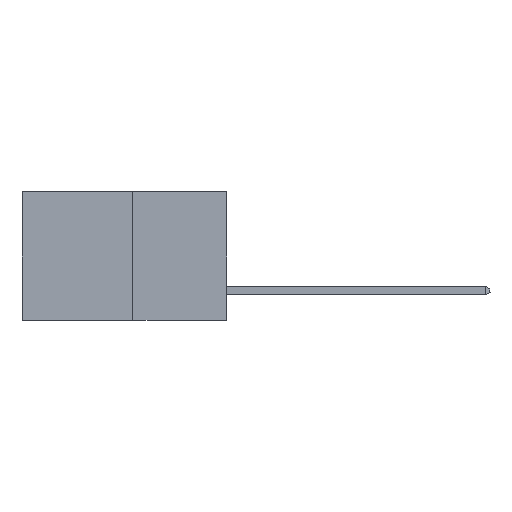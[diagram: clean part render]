
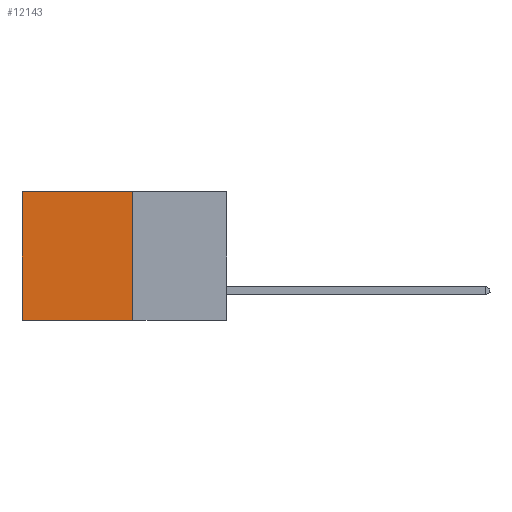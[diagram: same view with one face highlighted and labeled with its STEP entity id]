
A CAD part, left-side view. The second image highlights one B-rep face of the part: STEP entity #12143.
In plain terms, the highlighted planar face has unit normal (-1, 0, 0).
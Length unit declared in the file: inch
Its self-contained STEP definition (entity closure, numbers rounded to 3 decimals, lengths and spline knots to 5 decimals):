
#59 = ORIENTED_EDGE ( 'NONE', *, *, #7496, .T. ) ;
#542 = ORIENTED_EDGE ( 'NONE', *, *, #7257, .T. ) ;
#1475 = PLANE ( 'NONE',  #12065 ) ;
#1591 = CARTESIAN_POINT ( 'NONE',  ( 0.277, 0.27, 0. ) ) ;
#1652 = ORIENTED_EDGE ( 'NONE', *, *, #2605, .F. ) ;
#2120 = VERTEX_POINT ( 'NONE', #10665 ) ;
#2255 = VECTOR ( 'NONE', #6685, 39.37008 ) ;
#2542 = DIRECTION ( 'NONE',  ( 1., 0., 0. ) ) ;
#2605 = EDGE_CURVE ( 'NONE', #9794, #3217, #8461, .T. ) ;
#2678 = DIRECTION ( 'NONE',  ( 0., 1., 0. ) ) ;
#2694 = ORIENTED_EDGE ( 'NONE', *, *, #3458, .F. ) ;
#2736 = CARTESIAN_POINT ( 'NONE',  ( 0.277, 0.27, -0.37 ) ) ;
#2745 = VECTOR ( 'NONE', #10553, 39.37008 ) ;
#2899 = VECTOR ( 'NONE', #5490, 39.37008 ) ;
#3217 = VERTEX_POINT ( 'NONE', #6727 ) ;
#3458 = EDGE_CURVE ( 'NONE', #2120, #9794, #5282, .T. ) ;
#3579 = CARTESIAN_POINT ( 'NONE',  ( 0.277, 0.27, -0.37 ) ) ;
#5282 = LINE ( 'NONE', #11705, #2255 ) ;
#5490 = DIRECTION ( 'NONE',  ( 0., 0., -1. ) ) ;
#6559 = CARTESIAN_POINT ( 'NONE',  ( 0.277, 0.59, -0.37 ) ) ;
#6685 = DIRECTION ( 'NONE',  ( 0., 0., -1. ) ) ;
#6727 = CARTESIAN_POINT ( 'NONE',  ( 0.277, 0.59, -0.37 ) ) ;
#7257 = EDGE_CURVE ( 'NONE', #2120, #11512, #12178, .T. ) ;
#7467 = VECTOR ( 'NONE', #2678, 39.37008 ) ;
#7496 = EDGE_CURVE ( 'NONE', #11512, #3217, #10965, .T. ) ;
#7606 = CARTESIAN_POINT ( 'NONE',  ( 0.277, 0.59, 0. ) ) ;
#8461 = LINE ( 'NONE', #10872, #2745 ) ;
#9794 = VERTEX_POINT ( 'NONE', #2736 ) ;
#9806 = DIRECTION ( 'NONE',  ( 0., 0., -1. ) ) ;
#10553 = DIRECTION ( 'NONE',  ( 0., 1., 0. ) ) ;
#10665 = CARTESIAN_POINT ( 'NONE',  ( 0.277, 0.27, 0. ) ) ;
#10872 = CARTESIAN_POINT ( 'NONE',  ( 0.277, 0.27, -0.37 ) ) ;
#10965 = LINE ( 'NONE', #6559, #2899 ) ;
#11512 = VERTEX_POINT ( 'NONE', #7606 ) ;
#11705 = CARTESIAN_POINT ( 'NONE',  ( 0.277, 0.27, -0.37 ) ) ;
#11745 = FACE_OUTER_BOUND ( 'NONE', #12539, .T. ) ;
#12065 = AXIS2_PLACEMENT_3D ( 'NONE', #3579, #2542, #9806 ) ;
#12143 = ADVANCED_FACE ( 'NONE', ( #11745 ), #1475, .F. ) ;
#12178 = LINE ( 'NONE', #1591, #7467 ) ;
#12539 = EDGE_LOOP ( 'NONE', ( #59, #1652, #2694, #542 ) ) ;
